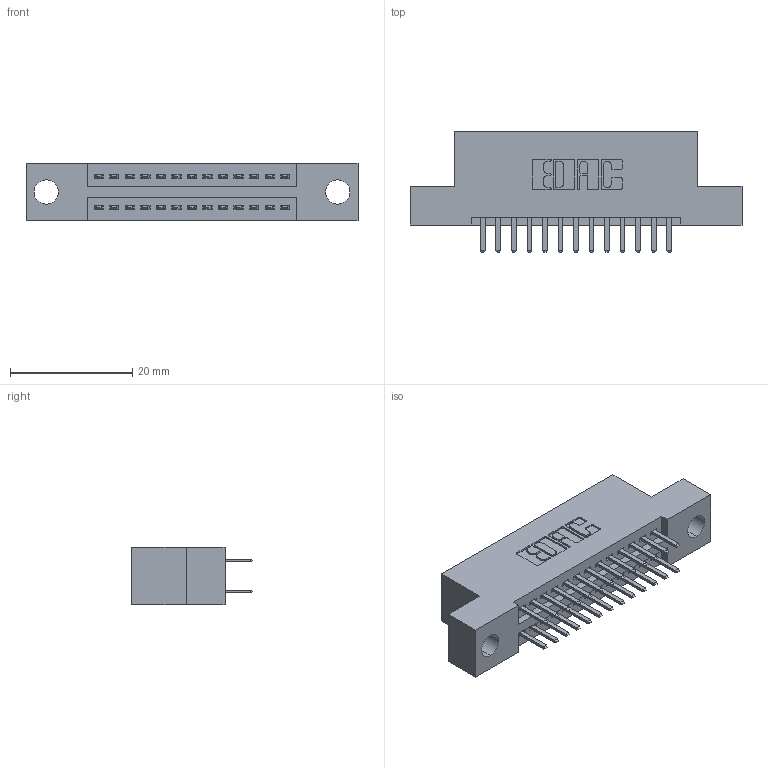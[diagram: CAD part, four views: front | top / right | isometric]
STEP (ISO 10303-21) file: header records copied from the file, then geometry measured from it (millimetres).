
FILE_DESCRIPTION (( 'STEP AP203' ), '1' );
FILE_NAME ('395-026-520-204.STEP', '2021-06-16T19:22:32', ( '' ), ( '' ), 'SwSTEP 2.0', 'SolidWorks 2020', '' );
FILE_SCHEMA (( 'CONFIG_CONTROL_DESIGN' ));
Length unit declared in the file: inch
Products named in the file (3): 345 Part_Flush Mounting Lugs - 0.156 Dia-TI; 345-292-001_345-293-120; 395-026-520-204
Assembly tree (27 placements, depth 2):
  395-026-520-204
    345 Part_Flush Mounting Lugs - 0.156 Dia-TI
    345-292-001_345-293-120  x26
Bounding box: 54.23 x 19.68 x 9.4 mm (x, y, z)
Volume: 4881.3 mm3; surface area: 6481 mm2
Topology: 27 solids, 27 shells, 1544 faces, 4459 edges, 2902 vertices
Faces by surface type: plane 1004, cylinder 540
Entity records: 14637 total; most frequent: CARTESIAN_POINT 2498, ORIENTED_EDGE 2418, DIRECTION 2225, EDGE_CURVE 1209, LINE 1021, VECTOR 1021, VERTEX_POINT 802, AXIS2_PLACEMENT_3D 602
